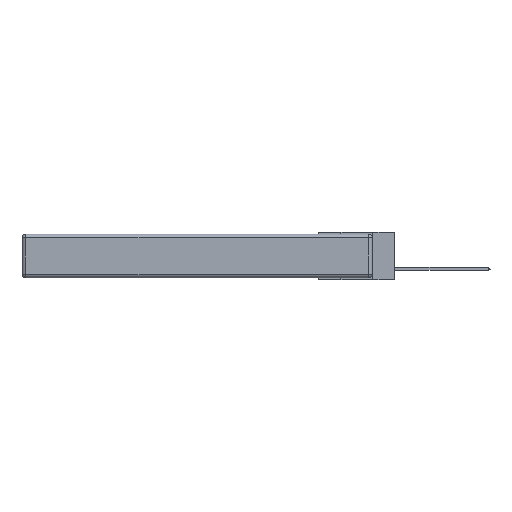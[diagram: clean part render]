
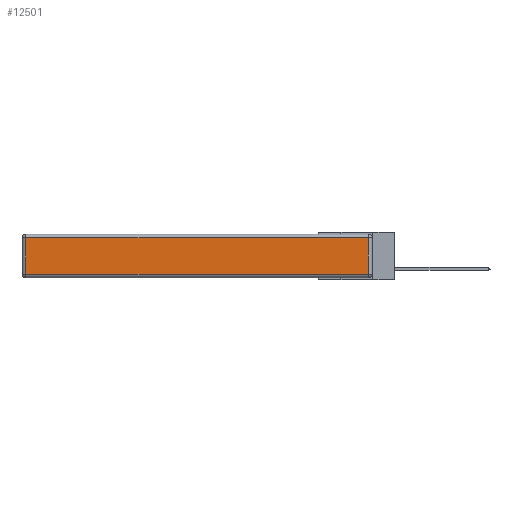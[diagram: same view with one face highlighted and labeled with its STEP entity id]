
A CAD part, left-side view. The second image highlights one B-rep face of the part: STEP entity #12501.
In plain terms, the highlighted planar face has unit normal (-1, 0, 0).
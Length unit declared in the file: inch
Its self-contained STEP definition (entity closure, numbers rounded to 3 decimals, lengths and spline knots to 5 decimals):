
#352 = CARTESIAN_POINT ( 'NONE',  ( 0., 0.03, -0.03 ) ) ;
#1122 = VECTOR ( 'NONE', #14782, 39.37008 ) ;
#1529 = VECTOR ( 'NONE', #2234, 39.37008 ) ;
#1797 = CARTESIAN_POINT ( 'NONE',  ( 0., 2.72, -0.343 ) ) ;
#1920 = CARTESIAN_POINT ( 'NONE',  ( 0., 0., -0.313 ) ) ;
#2064 = LINE ( 'NONE', #1797, #11408 ) ;
#2234 = DIRECTION ( 'NONE',  ( 0., 1., 0. ) ) ;
#2328 = EDGE_LOOP ( 'NONE', ( #14245, #7018, #10488, #11570 ) ) ;
#2507 = CARTESIAN_POINT ( 'NONE',  ( 0., 2.72, -0.03 ) ) ;
#2520 = FACE_OUTER_BOUND ( 'NONE', #2328, .T. ) ;
#2698 = AXIS2_PLACEMENT_3D ( 'NONE', #13286, #3920, #9879 ) ;
#3920 = DIRECTION ( 'NONE',  ( -1., 0., 0. ) ) ;
#4030 = CARTESIAN_POINT ( 'NONE',  ( 0., 2.72, -0.313 ) ) ;
#4488 = CARTESIAN_POINT ( 'NONE',  ( 0., 0.03, -0.343 ) ) ;
#6156 = LINE ( 'NONE', #4488, #12210 ) ;
#6856 = EDGE_CURVE ( 'NONE', #7395, #7095, #13913, .T. ) ;
#7018 = ORIENTED_EDGE ( 'NONE', *, *, #13416, .T. ) ;
#7095 = VERTEX_POINT ( 'NONE', #2507 ) ;
#7266 = LINE ( 'NONE', #1920, #1122 ) ;
#7395 = VERTEX_POINT ( 'NONE', #352 ) ;
#8739 = DIRECTION ( 'NONE',  ( 0., 0., -1. ) ) ;
#9879 = DIRECTION ( 'NONE',  ( 0., 0., 1. ) ) ;
#10312 = DIRECTION ( 'NONE',  ( 0., 0., 1. ) ) ;
#10467 = EDGE_CURVE ( 'NONE', #7095, #14051, #2064, .T. ) ;
#10488 = ORIENTED_EDGE ( 'NONE', *, *, #6856, .T. ) ;
#10974 = PLANE ( 'NONE',  #2698 ) ;
#11408 = VECTOR ( 'NONE', #8739, 39.37008 ) ;
#11501 = VERTEX_POINT ( 'NONE', #14816 ) ;
#11570 = ORIENTED_EDGE ( 'NONE', *, *, #10467, .T. ) ;
#12210 = VECTOR ( 'NONE', #10312, 39.37008 ) ;
#12501 = ADVANCED_FACE ( 'NONE', ( #2520 ), #10974, .T. ) ;
#12763 = EDGE_CURVE ( 'NONE', #14051, #11501, #7266, .T. ) ;
#13286 = CARTESIAN_POINT ( 'NONE',  ( 0., 0., -0.343 ) ) ;
#13416 = EDGE_CURVE ( 'NONE', #11501, #7395, #6156, .T. ) ;
#13767 = CARTESIAN_POINT ( 'NONE',  ( 0., 2.75, -0.03 ) ) ;
#13913 = LINE ( 'NONE', #13767, #1529 ) ;
#14051 = VERTEX_POINT ( 'NONE', #4030 ) ;
#14245 = ORIENTED_EDGE ( 'NONE', *, *, #12763, .T. ) ;
#14782 = DIRECTION ( 'NONE',  ( 0., -1., 0. ) ) ;
#14816 = CARTESIAN_POINT ( 'NONE',  ( 0., 0.03, -0.313 ) ) ;
